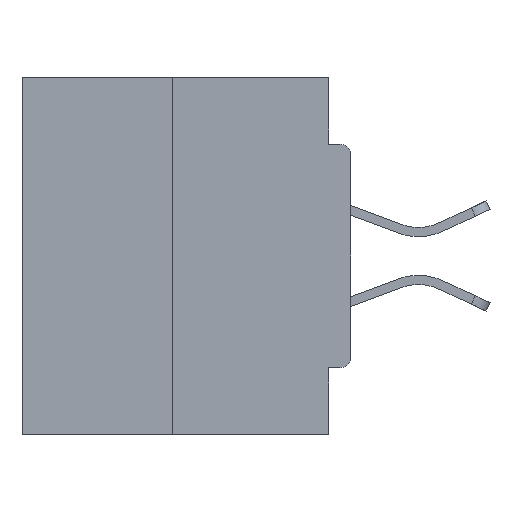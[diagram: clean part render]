
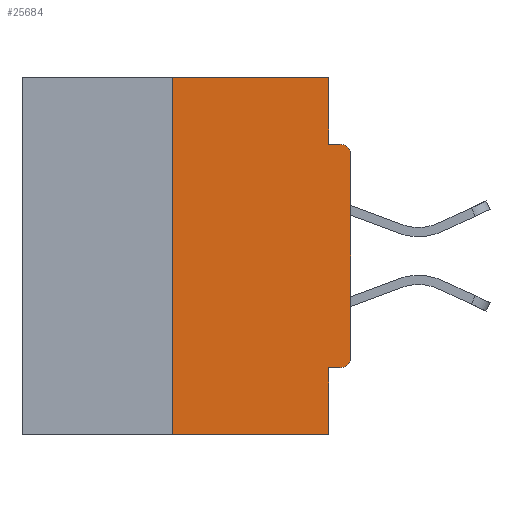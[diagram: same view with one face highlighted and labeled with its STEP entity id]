
A CAD part, left-side view. The second image highlights one B-rep face of the part: STEP entity #25684.
In plain terms, the highlighted planar face has unit normal (-1, 0, 0).
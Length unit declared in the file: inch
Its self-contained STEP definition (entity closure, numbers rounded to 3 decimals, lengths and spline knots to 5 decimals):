
#57 = VECTOR ( 'NONE', #26988, 39.37008 ) ;
#181 = VECTOR ( 'NONE', #31647, 39.37008 ) ;
#193 = VERTEX_POINT ( 'NONE', #18009 ) ;
#395 = VERTEX_POINT ( 'NONE', #18841 ) ;
#409 = DIRECTION ( 'NONE',  ( 0., 0., -1. ) ) ;
#1143 = CARTESIAN_POINT ( 'NONE',  ( 0., 0., -0.4065 ) ) ;
#1695 = AXIS2_PLACEMENT_3D ( 'NONE', #5409, #5187, #409 ) ;
#2179 = ORIENTED_EDGE ( 'NONE', *, *, #17624, .T. ) ;
#2227 = EDGE_CURVE ( 'NONE', #193, #6190, #29660, .T. ) ;
#2575 = VERTEX_POINT ( 'NONE', #16473 ) ;
#3083 = CARTESIAN_POINT ( 'NONE',  ( 0., 0.031, -0.5 ) ) ;
#3609 = VECTOR ( 'NONE', #26862, 39.37008 ) ;
#3888 = VECTOR ( 'NONE', #11316, 39.37008 ) ;
#4016 = ORIENTED_EDGE ( 'NONE', *, *, #24061, .F. ) ;
#4462 = LINE ( 'NONE', #28140, #20388 ) ;
#5187 = DIRECTION ( 'NONE',  ( 1., 0., 0. ) ) ;
#5409 = CARTESIAN_POINT ( 'NONE',  ( 0., 0.46, 0. ) ) ;
#6190 = VERTEX_POINT ( 'NONE', #23998 ) ;
#8215 = VERTEX_POINT ( 'NONE', #13151 ) ;
#8219 = DIRECTION ( 'NONE',  ( 0., 0., 1. ) ) ;
#8400 = EDGE_CURVE ( 'NONE', #20859, #30588, #15926, .T. ) ;
#9112 = CARTESIAN_POINT ( 'NONE',  ( 0., 0.031, -0.0935 ) ) ;
#9433 = FACE_OUTER_BOUND ( 'NONE', #15910, .T. ) ;
#10005 = CARTESIAN_POINT ( 'NONE',  ( 0., 0.46, -0.5 ) ) ;
#10039 = ORIENTED_EDGE ( 'NONE', *, *, #8400, .T. ) ;
#10584 = CARTESIAN_POINT ( 'NONE',  ( 0., 0., -0.0935 ) ) ;
#10850 = VERTEX_POINT ( 'NONE', #29229 ) ;
#11316 = DIRECTION ( 'NONE',  ( 0., 0., 1. ) ) ;
#11326 = DIRECTION ( 'NONE',  ( -1., 0., 0. ) ) ;
#11976 = CIRCLE ( 'NONE', #28561, 0.015 ) ;
#12146 = CARTESIAN_POINT ( 'NONE',  ( 0., 0.015, -0.0935 ) ) ;
#13151 = CARTESIAN_POINT ( 'NONE',  ( 0., 0., -0.3915 ) ) ;
#13180 = DIRECTION ( 'NONE',  ( -1., 0., 0. ) ) ;
#13550 = VERTEX_POINT ( 'NONE', #9112 ) ;
#13672 = ORIENTED_EDGE ( 'NONE', *, *, #25549, .F. ) ;
#13823 = CARTESIAN_POINT ( 'NONE',  ( 0., 0.015, -0.4065 ) ) ;
#14039 = DIRECTION ( 'NONE',  ( 0., 1., 0. ) ) ;
#14115 = VECTOR ( 'NONE', #30223, 39.37008 ) ;
#14340 = EDGE_CURVE ( 'NONE', #2575, #6190, #21017, .T. ) ;
#14546 = EDGE_CURVE ( 'NONE', #193, #10850, #15541, .T. ) ;
#15269 = PLANE ( 'NONE',  #1695 ) ;
#15541 = LINE ( 'NONE', #31255, #3888 ) ;
#15910 = EDGE_LOOP ( 'NONE', ( #19217, #22386, #23766, #25214, #26006, #18756, #2179, #10039, #4016, #13672 ) ) ;
#15926 = CIRCLE ( 'NONE', #23414, 0.015 ) ;
#16473 = CARTESIAN_POINT ( 'NONE',  ( 0., 0.031, -0.4065 ) ) ;
#17181 = EDGE_CURVE ( 'NONE', #10850, #395, #28626, .T. ) ;
#17624 = EDGE_CURVE ( 'NONE', #8215, #20859, #4462, .T. ) ;
#18009 = CARTESIAN_POINT ( 'NONE',  ( 0., 0.25, -0.5 ) ) ;
#18079 = DIRECTION ( 'NONE',  ( 0., 0., -1. ) ) ;
#18756 = ORIENTED_EDGE ( 'NONE', *, *, #31615, .T. ) ;
#18762 = CARTESIAN_POINT ( 'NONE',  ( 0., 0.46, 0. ) ) ;
#18796 = CARTESIAN_POINT ( 'NONE',  ( 0., 0., -0.1085 ) ) ;
#18806 = CARTESIAN_POINT ( 'NONE',  ( 0., 0.015, -0.3915 ) ) ;
#18841 = CARTESIAN_POINT ( 'NONE',  ( 0., 0.031, 0. ) ) ;
#19158 = LINE ( 'NONE', #22050, #3609 ) ;
#19217 = ORIENTED_EDGE ( 'NONE', *, *, #17181, .F. ) ;
#19248 = DIRECTION ( 'NONE',  ( 0., 0., -1. ) ) ;
#20388 = VECTOR ( 'NONE', #8219, 39.37008 ) ;
#20714 = VECTOR ( 'NONE', #14039, 39.37008 ) ;
#20784 = LINE ( 'NONE', #10584, #14115 ) ;
#20859 = VERTEX_POINT ( 'NONE', #18796 ) ;
#21017 = LINE ( 'NONE', #3083, #26480 ) ;
#22050 = CARTESIAN_POINT ( 'NONE',  ( 0., 0.031, 0. ) ) ;
#22386 = ORIENTED_EDGE ( 'NONE', *, *, #14546, .F. ) ;
#22782 = VERTEX_POINT ( 'NONE', #13823 ) ;
#23414 = AXIS2_PLACEMENT_3D ( 'NONE', #30744, #13180, #18079 ) ;
#23766 = ORIENTED_EDGE ( 'NONE', *, *, #2227, .T. ) ;
#23840 = LINE ( 'NONE', #1143, #20714 ) ;
#23998 = CARTESIAN_POINT ( 'NONE',  ( 0., 0.031, -0.5 ) ) ;
#24061 = EDGE_CURVE ( 'NONE', #13550, #30588, #20784, .T. ) ;
#25214 = ORIENTED_EDGE ( 'NONE', *, *, #14340, .F. ) ;
#25549 = EDGE_CURVE ( 'NONE', #395, #13550, #19158, .T. ) ;
#25684 = ADVANCED_FACE ( 'NONE', ( #9433 ), #15269, .F. ) ;
#25948 = EDGE_CURVE ( 'NONE', #22782, #2575, #23840, .T. ) ;
#26006 = ORIENTED_EDGE ( 'NONE', *, *, #25948, .F. ) ;
#26480 = VECTOR ( 'NONE', #27778, 39.37008 ) ;
#26862 = DIRECTION ( 'NONE',  ( 0., 0., -1. ) ) ;
#26988 = DIRECTION ( 'NONE',  ( 0., -1., 0. ) ) ;
#27778 = DIRECTION ( 'NONE',  ( 0., 0., -1. ) ) ;
#28140 = CARTESIAN_POINT ( 'NONE',  ( 0., 0., 0. ) ) ;
#28561 = AXIS2_PLACEMENT_3D ( 'NONE', #18806, #11326, #19248 ) ;
#28626 = LINE ( 'NONE', #18762, #181 ) ;
#29229 = CARTESIAN_POINT ( 'NONE',  ( 0., 0.25, 0. ) ) ;
#29660 = LINE ( 'NONE', #10005, #57 ) ;
#30223 = DIRECTION ( 'NONE',  ( 0., -1., 0. ) ) ;
#30588 = VERTEX_POINT ( 'NONE', #12146 ) ;
#30744 = CARTESIAN_POINT ( 'NONE',  ( 0., 0.015, -0.1085 ) ) ;
#31255 = CARTESIAN_POINT ( 'NONE',  ( 0., 0.25, 0. ) ) ;
#31615 = EDGE_CURVE ( 'NONE', #22782, #8215, #11976, .T. ) ;
#31647 = DIRECTION ( 'NONE',  ( 0., -1., 0. ) ) ;
